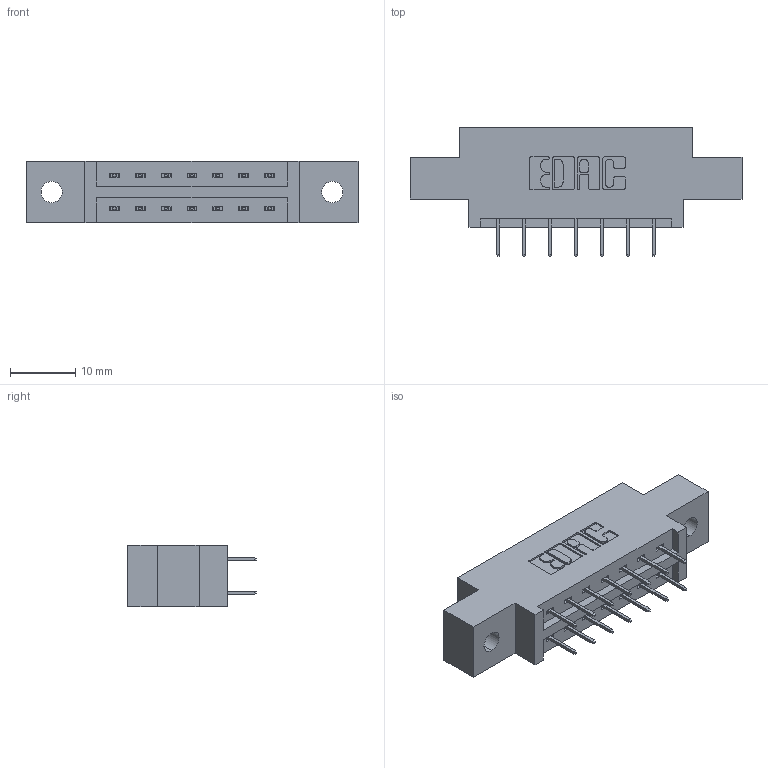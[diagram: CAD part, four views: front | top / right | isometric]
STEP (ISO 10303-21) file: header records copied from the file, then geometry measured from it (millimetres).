
FILE_DESCRIPTION (( 'STEP AP203' ), '1' );
FILE_NAME ('337-014-524-802.STEP', '2018-08-04T14:37:43', ( '' ), ( '' ), 'SwSTEP 2.0', 'SolidWorks 2016', '' );
FILE_SCHEMA (( 'CONFIG_CONTROL_DESIGN' ));
Length unit declared in the file: inch
Products named in the file (3): 345-292-001_345-293-124; 337-014-524-802; 337 Part_0.170 Offset - 0.128 Dia
Assembly tree (15 placements, depth 2):
  337-014-524-802
    337 Part_0.170 Offset - 0.128 Dia
    345-292-001_345-293-124  x14
Bounding box: 50.75 x 19.69 x 9.4 mm (x, y, z)
Volume: 4707.1 mm3; surface area: 4750.9 mm2
Topology: 15 solids, 15 shells, 930 faces, 2633 edges, 1698 vertices
Faces by surface type: plane 690, cylinder 240
Entity records: 10163 total; most frequent: CARTESIAN_POINT 1742, ORIENTED_EDGE 1678, DIRECTION 1547, EDGE_CURVE 839, LINE 715, VECTOR 715, VERTEX_POINT 554, AXIS2_PLACEMENT_3D 416
